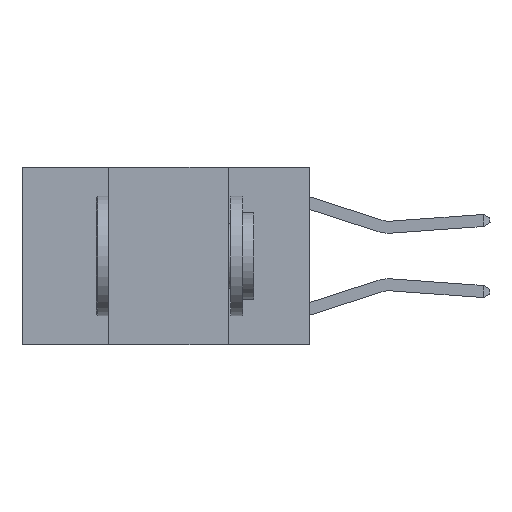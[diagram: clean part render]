
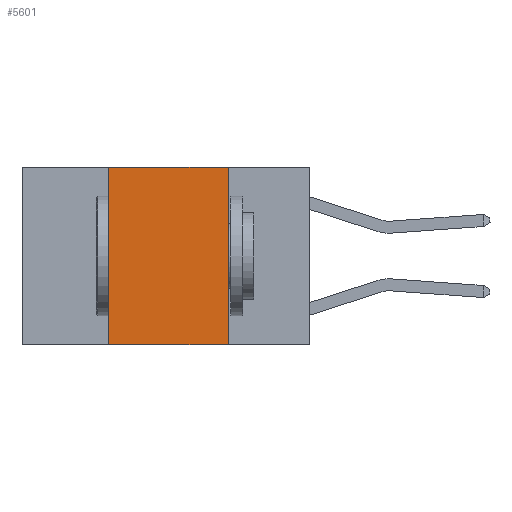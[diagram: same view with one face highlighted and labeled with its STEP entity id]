
A CAD part, left-side view. The second image highlights one B-rep face of the part: STEP entity #5601.
In plain terms, the highlighted planar face has unit normal (-1, 0, 0).
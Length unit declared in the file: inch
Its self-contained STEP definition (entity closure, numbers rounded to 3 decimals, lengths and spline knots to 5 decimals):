
#169 = DIRECTION ( 'NONE',  ( 0., -1., 0. ) ) ;
#646 = FACE_OUTER_BOUND ( 'NONE', #3744, .T. ) ;
#1037 = VECTOR ( 'NONE', #9159, 39.37008 ) ;
#1493 = VERTEX_POINT ( 'NONE', #4383 ) ;
#1680 = VECTOR ( 'NONE', #5667, 39.37008 ) ;
#2252 = DIRECTION ( 'NONE',  ( 1., 0., 0. ) ) ;
#2903 = VECTOR ( 'NONE', #7821, 39.37008 ) ;
#2944 = AXIS2_PLACEMENT_3D ( 'NONE', #9891, #2252, #7624 ) ;
#2970 = EDGE_CURVE ( 'NONE', #9656, #5223, #3790, .T. ) ;
#3043 = ORIENTED_EDGE ( 'NONE', *, *, #3259, .F. ) ;
#3259 = EDGE_CURVE ( 'NONE', #9135, #9656, #6986, .T. ) ;
#3617 = VECTOR ( 'NONE', #169, 39.37008 ) ;
#3691 = CARTESIAN_POINT ( 'NONE',  ( 0., 0.17, 0. ) ) ;
#3744 = EDGE_LOOP ( 'NONE', ( #5355, #3043, #5131, #4887 ) ) ;
#3790 = LINE ( 'NONE', #6665, #1680 ) ;
#4383 = CARTESIAN_POINT ( 'NONE',  ( 0., 0.42, -0.37 ) ) ;
#4555 = EDGE_CURVE ( 'NONE', #1493, #5223, #5671, .T. ) ;
#4887 = ORIENTED_EDGE ( 'NONE', *, *, #4555, .T. ) ;
#5131 = ORIENTED_EDGE ( 'NONE', *, *, #6294, .F. ) ;
#5223 = VERTEX_POINT ( 'NONE', #5670 ) ;
#5355 = ORIENTED_EDGE ( 'NONE', *, *, #2970, .F. ) ;
#5601 = ADVANCED_FACE ( 'NONE', ( #646 ), #6883, .F. ) ;
#5667 = DIRECTION ( 'NONE',  ( 0., 0., -1. ) ) ;
#5670 = CARTESIAN_POINT ( 'NONE',  ( 0., 0.17, -0.37 ) ) ;
#5671 = LINE ( 'NONE', #9408, #3617 ) ;
#5946 = CARTESIAN_POINT ( 'NONE',  ( 0., 0.42, 0. ) ) ;
#6156 = CARTESIAN_POINT ( 'NONE',  ( 0., 0.42, 0. ) ) ;
#6294 = EDGE_CURVE ( 'NONE', #1493, #9135, #8743, .T. ) ;
#6665 = CARTESIAN_POINT ( 'NONE',  ( 0., 0.17, 0. ) ) ;
#6883 = PLANE ( 'NONE',  #2944 ) ;
#6986 = LINE ( 'NONE', #8058, #2903 ) ;
#7624 = DIRECTION ( 'NONE',  ( 0., 0., -1. ) ) ;
#7821 = DIRECTION ( 'NONE',  ( 0., -1., 0. ) ) ;
#8058 = CARTESIAN_POINT ( 'NONE',  ( 0., 0.6, 0. ) ) ;
#8743 = LINE ( 'NONE', #6156, #1037 ) ;
#9135 = VERTEX_POINT ( 'NONE', #5946 ) ;
#9159 = DIRECTION ( 'NONE',  ( 0., 0., 1. ) ) ;
#9408 = CARTESIAN_POINT ( 'NONE',  ( 0., 0.6, -0.37 ) ) ;
#9656 = VERTEX_POINT ( 'NONE', #3691 ) ;
#9891 = CARTESIAN_POINT ( 'NONE',  ( 0., 0.6, 0. ) ) ;
